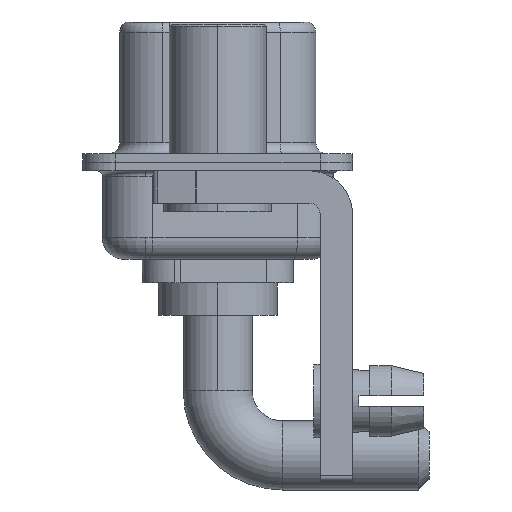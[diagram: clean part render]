
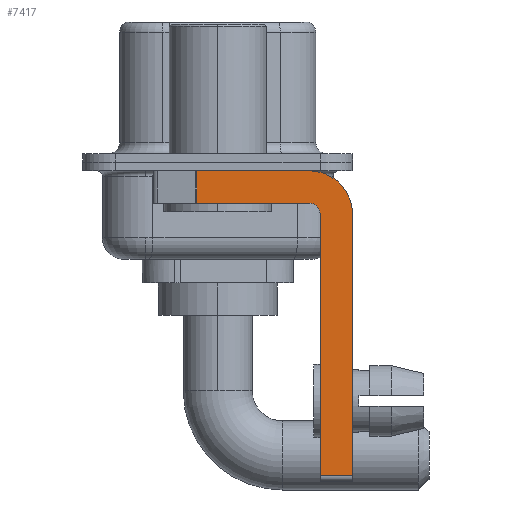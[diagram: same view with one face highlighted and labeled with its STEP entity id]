
A CAD part, left-side view. The second image highlights one B-rep face of the part: STEP entity #7417.
In plain terms, the highlighted planar face has unit normal (-1, 0, 0).
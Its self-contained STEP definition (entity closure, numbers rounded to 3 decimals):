
#553 = VECTOR ( 'NONE', #4077, 1000. ) ;
#692 = CARTESIAN_POINT ( 'NONE',  ( -2.9, -4.25, -2.4 ) ) ;
#872 = VECTOR ( 'NONE', #7753, 1000. ) ;
#972 = CARTESIAN_POINT ( 'NONE',  ( -2.9, -4.25, -14.55 ) ) ;
#1494 = FACE_OUTER_BOUND ( 'NONE', #17320, .T. ) ;
#1747 = ORIENTED_EDGE ( 'NONE', *, *, #18759, .F. ) ;
#2285 = CARTESIAN_POINT ( 'NONE',  ( -2.9, -4.75, -14.55 ) ) ;
#2357 = ORIENTED_EDGE ( 'NONE', *, *, #8143, .F. ) ;
#2709 = VERTEX_POINT ( 'NONE', #8029 ) ;
#3226 = EDGE_CURVE ( 'NONE', #3534, #18622, #18397, .T. ) ;
#3534 = VERTEX_POINT ( 'NONE', #6277 ) ;
#3582 = DIRECTION ( 'NONE',  ( 0., -1., 0. ) ) ;
#3807 = DIRECTION ( 'NONE',  ( -1., 0., 0. ) ) ;
#3903 = VECTOR ( 'NONE', #11147, 1000. ) ;
#3931 = AXIS2_PLACEMENT_3D ( 'NONE', #12229, #16433, #18354 ) ;
#4077 = DIRECTION ( 'NONE',  ( 0., 0., -1. ) ) ;
#4533 = LINE ( 'NONE', #7517, #14011 ) ;
#4769 = LINE ( 'NONE', #9822, #872 ) ;
#4999 = DIRECTION ( 'NONE',  ( 1., 0., 0. ) ) ;
#5434 = EDGE_CURVE ( 'NONE', #12442, #15925, #17574, .T. ) ;
#6277 = CARTESIAN_POINT ( 'NONE',  ( -2.9, -4.25, -0.4 ) ) ;
#6471 = CARTESIAN_POINT ( 'NONE',  ( -2.9, 0.978, -1.9 ) ) ;
#6479 = CARTESIAN_POINT ( 'NONE',  ( -2.9, -6.25, -2.4 ) ) ;
#7417 = ADVANCED_FACE ( 'NONE', ( #1494 ), #13452, .F. ) ;
#7517 = CARTESIAN_POINT ( 'NONE',  ( -2.9, 0.978, -1.9 ) ) ;
#7753 = DIRECTION ( 'NONE',  ( 0., -1., 0. ) ) ;
#8029 = CARTESIAN_POINT ( 'NONE',  ( -2.9, -4.75, -2.4 ) ) ;
#8143 = EDGE_CURVE ( 'NONE', #19092, #2709, #15861, .T. ) ;
#8403 = DIRECTION ( 'NONE',  ( 0., 0., 1. ) ) ;
#9260 = VERTEX_POINT ( 'NONE', #13815 ) ;
#9434 = VECTOR ( 'NONE', #3582, 1000. ) ;
#9702 = CARTESIAN_POINT ( 'NONE',  ( -2.9, -4.25, -1.9 ) ) ;
#9822 = CARTESIAN_POINT ( 'NONE',  ( -2.9, 3., -0.4 ) ) ;
#10865 = ORIENTED_EDGE ( 'NONE', *, *, #3226, .F. ) ;
#10914 = ORIENTED_EDGE ( 'NONE', *, *, #12977, .T. ) ;
#11147 = DIRECTION ( 'NONE',  ( 0., 0., 1. ) ) ;
#11231 = ORIENTED_EDGE ( 'NONE', *, *, #16365, .F. ) ;
#11631 = CARTESIAN_POINT ( 'NONE',  ( -2.9, -4.25, -1.9 ) ) ;
#11790 = CARTESIAN_POINT ( 'NONE',  ( -2.9, -6.25, -2.4 ) ) ;
#12229 = CARTESIAN_POINT ( 'NONE',  ( -2.9, -4.25, -2.4 ) ) ;
#12442 = VERTEX_POINT ( 'NONE', #9702 ) ;
#12578 = EDGE_CURVE ( 'NONE', #2709, #12442, #19374, .T. ) ;
#12666 = AXIS2_PLACEMENT_3D ( 'NONE', #692, #3807, #8403 ) ;
#12977 = EDGE_CURVE ( 'NONE', #19092, #18914, #15909, .T. ) ;
#13017 = ORIENTED_EDGE ( 'NONE', *, *, #5434, .F. ) ;
#13452 = PLANE ( 'NONE',  #3931 ) ;
#13815 = CARTESIAN_POINT ( 'NONE',  ( -2.9, 0.978, -0.4 ) ) ;
#13976 = VECTOR ( 'NONE', #17756, 1000. ) ;
#14011 = VECTOR ( 'NONE', #15436, 1000. ) ;
#14499 = LINE ( 'NONE', #11790, #553 ) ;
#15115 = ORIENTED_EDGE ( 'NONE', *, *, #12578, .F. ) ;
#15198 = CARTESIAN_POINT ( 'NONE',  ( -2.9, -6.25, -14.55 ) ) ;
#15436 = DIRECTION ( 'NONE',  ( 0., 0., -1. ) ) ;
#15861 = LINE ( 'NONE', #18890, #3903 ) ;
#15909 = LINE ( 'NONE', #972, #9434 ) ;
#15919 = DIRECTION ( 'NONE',  ( 0., 0., -1. ) ) ;
#15925 = VERTEX_POINT ( 'NONE', #6471 ) ;
#16365 = EDGE_CURVE ( 'NONE', #9260, #3534, #4769, .T. ) ;
#16433 = DIRECTION ( 'NONE',  ( 1., 0., 0. ) ) ;
#16696 = EDGE_CURVE ( 'NONE', #9260, #15925, #4533, .T. ) ;
#17320 = EDGE_LOOP ( 'NONE', ( #11231, #17921, #13017, #15115, #2357, #10914, #1747, #10865 ) ) ;
#17574 = LINE ( 'NONE', #11631, #13976 ) ;
#17756 = DIRECTION ( 'NONE',  ( 0., 1., 0. ) ) ;
#17921 = ORIENTED_EDGE ( 'NONE', *, *, #16696, .T. ) ;
#18354 = DIRECTION ( 'NONE',  ( 0., 0., -1. ) ) ;
#18397 = CIRCLE ( 'NONE', #19351, 2. ) ;
#18622 = VERTEX_POINT ( 'NONE', #6479 ) ;
#18759 = EDGE_CURVE ( 'NONE', #18622, #18914, #14499, .T. ) ;
#18890 = CARTESIAN_POINT ( 'NONE',  ( -2.9, -4.75, -14.8 ) ) ;
#18914 = VERTEX_POINT ( 'NONE', #15198 ) ;
#19028 = CARTESIAN_POINT ( 'NONE',  ( -2.9, -4.25, -2.4 ) ) ;
#19092 = VERTEX_POINT ( 'NONE', #2285 ) ;
#19351 = AXIS2_PLACEMENT_3D ( 'NONE', #19028, #4999, #15919 ) ;
#19374 = CIRCLE ( 'NONE', #12666, 0.5 ) ;
